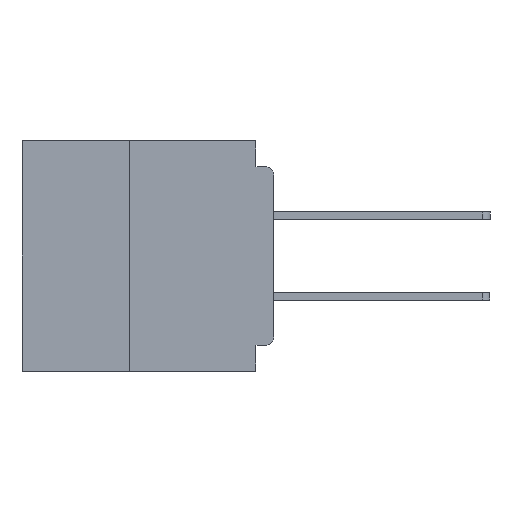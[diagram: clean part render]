
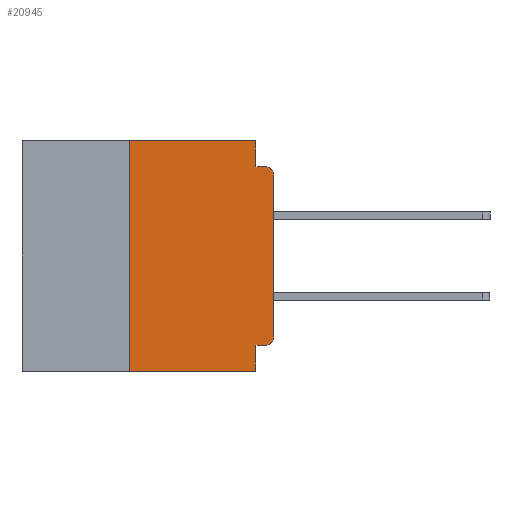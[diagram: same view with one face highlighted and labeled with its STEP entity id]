
A CAD part, left-side view. The second image highlights one B-rep face of the part: STEP entity #20945.
In plain terms, the highlighted planar face has unit normal (-1, 0, 0).
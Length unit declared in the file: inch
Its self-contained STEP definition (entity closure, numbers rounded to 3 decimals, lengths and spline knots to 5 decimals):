
#348 = CARTESIAN_POINT ( 'NONE',  ( 0., 0.25, -0.4 ) ) ;
#2660 = VECTOR ( 'NONE', #12221, 39.37008 ) ;
#2990 = EDGE_LOOP ( 'NONE', ( #30418, #12050, #26791, #27463, #31308, #37348, #7928, #6343, #39299, #18550 ) ) ;
#4067 = CARTESIAN_POINT ( 'NONE',  ( 0., 0., 0. ) ) ;
#4201 = AXIS2_PLACEMENT_3D ( 'NONE', #30078, #10522, #33375 ) ;
#5072 = CARTESIAN_POINT ( 'NONE',  ( 0., 0.437, 0. ) ) ;
#6161 = EDGE_CURVE ( 'NONE', #16101, #41000, #12043, .T. ) ;
#6162 = VECTOR ( 'NONE', #20634, 39.37008 ) ;
#6343 = ORIENTED_EDGE ( 'NONE', *, *, #12228, .F. ) ;
#6847 = VECTOR ( 'NONE', #16780, 39.37008 ) ;
#6880 = DIRECTION ( 'NONE',  ( 1., 0., 0. ) ) ;
#7031 = CARTESIAN_POINT ( 'NONE',  ( 0., 0.031, 0. ) ) ;
#7182 = EDGE_CURVE ( 'NONE', #24444, #38639, #15529, .T. ) ;
#7481 = VERTEX_POINT ( 'NONE', #21600 ) ;
#7928 = ORIENTED_EDGE ( 'NONE', *, *, #39443, .T. ) ;
#7967 = EDGE_CURVE ( 'NONE', #38639, #18185, #24130, .T. ) ;
#9271 = DIRECTION ( 'NONE',  ( -1., 0., 0. ) ) ;
#10268 = CIRCLE ( 'NONE', #4201, 0.015 ) ;
#10323 = DIRECTION ( 'NONE',  ( 0., 0., -1. ) ) ;
#10348 = LINE ( 'NONE', #31800, #2660 ) ;
#10522 = DIRECTION ( 'NONE',  ( -1., 0., 0. ) ) ;
#11561 = VERTEX_POINT ( 'NONE', #23038 ) ;
#12043 = LINE ( 'NONE', #14273, #30445 ) ;
#12050 = ORIENTED_EDGE ( 'NONE', *, *, #19523, .T. ) ;
#12221 = DIRECTION ( 'NONE',  ( 0., -1., 0. ) ) ;
#12228 = EDGE_CURVE ( 'NONE', #41000, #37942, #25846, .T. ) ;
#14273 = CARTESIAN_POINT ( 'NONE',  ( 0., 0., -0.355 ) ) ;
#15447 = VECTOR ( 'NONE', #27931, 39.37008 ) ;
#15529 = LINE ( 'NONE', #348, #6847 ) ;
#16101 = VERTEX_POINT ( 'NONE', #27505 ) ;
#16662 = AXIS2_PLACEMENT_3D ( 'NONE', #28851, #9271, #32152 ) ;
#16780 = DIRECTION ( 'NONE',  ( 0., 0., 1. ) ) ;
#16905 = VECTOR ( 'NONE', #10323, 39.37008 ) ;
#17351 = DIRECTION ( 'NONE',  ( 0., 0., 1. ) ) ;
#17408 = CARTESIAN_POINT ( 'NONE',  ( 0., 0.031, -0.355 ) ) ;
#18185 = VERTEX_POINT ( 'NONE', #19617 ) ;
#18550 = ORIENTED_EDGE ( 'NONE', *, *, #36495, .T. ) ;
#18929 = LINE ( 'NONE', #7031, #16905 ) ;
#19523 = EDGE_CURVE ( 'NONE', #22600, #7481, #39201, .T. ) ;
#19617 = CARTESIAN_POINT ( 'NONE',  ( 0., 0.031, 0. ) ) ;
#20634 = DIRECTION ( 'NONE',  ( 0., -1., 0. ) ) ;
#20945 = ADVANCED_FACE ( 'NONE', ( #34033 ), #36154, .F. ) ;
#21600 = CARTESIAN_POINT ( 'NONE',  ( 0., 0.015, -0.045 ) ) ;
#21919 = AXIS2_PLACEMENT_3D ( 'NONE', #39435, #6880, #29736 ) ;
#22600 = VERTEX_POINT ( 'NONE', #33522 ) ;
#23038 = CARTESIAN_POINT ( 'NONE',  ( 0., 0.031, -0.045 ) ) ;
#23089 = VERTEX_POINT ( 'NONE', #39040 ) ;
#23923 = CARTESIAN_POINT ( 'NONE',  ( 0., 0., -0.045 ) ) ;
#24130 = LINE ( 'NONE', #5072, #15447 ) ;
#24418 = CARTESIAN_POINT ( 'NONE',  ( 0., 0.25, 0. ) ) ;
#24444 = VERTEX_POINT ( 'NONE', #30228 ) ;
#25825 = LINE ( 'NONE', #4067, #41150 ) ;
#25846 = LINE ( 'NONE', #29852, #42188 ) ;
#26575 = DIRECTION ( 'NONE',  ( 0., 0., -1. ) ) ;
#26791 = ORIENTED_EDGE ( 'NONE', *, *, #36557, .F. ) ;
#27463 = ORIENTED_EDGE ( 'NONE', *, *, #40379, .F. ) ;
#27505 = CARTESIAN_POINT ( 'NONE',  ( 0., 0.015, -0.355 ) ) ;
#27931 = DIRECTION ( 'NONE',  ( 0., -1., 0. ) ) ;
#28851 = CARTESIAN_POINT ( 'NONE',  ( 0., 0.015, -0.06 ) ) ;
#29736 = DIRECTION ( 'NONE',  ( 0., 0., -1. ) ) ;
#29852 = CARTESIAN_POINT ( 'NONE',  ( 0., 0.031, -0.4 ) ) ;
#30078 = CARTESIAN_POINT ( 'NONE',  ( 0., 0.015, -0.34 ) ) ;
#30228 = CARTESIAN_POINT ( 'NONE',  ( 0., 0.25, -0.4 ) ) ;
#30418 = ORIENTED_EDGE ( 'NONE', *, *, #33875, .T. ) ;
#30445 = VECTOR ( 'NONE', #37121, 39.37008 ) ;
#31308 = ORIENTED_EDGE ( 'NONE', *, *, #7967, .F. ) ;
#31800 = CARTESIAN_POINT ( 'NONE',  ( 0., 0.437, -0.4 ) ) ;
#32152 = DIRECTION ( 'NONE',  ( 0., 0., -1. ) ) ;
#33375 = DIRECTION ( 'NONE',  ( 0., 0., -1. ) ) ;
#33522 = CARTESIAN_POINT ( 'NONE',  ( 0., 0., -0.06 ) ) ;
#33875 = EDGE_CURVE ( 'NONE', #23089, #22600, #25825, .T. ) ;
#34033 = FACE_OUTER_BOUND ( 'NONE', #2990, .T. ) ;
#36154 = PLANE ( 'NONE',  #21919 ) ;
#36495 = EDGE_CURVE ( 'NONE', #16101, #23089, #10268, .T. ) ;
#36557 = EDGE_CURVE ( 'NONE', #11561, #7481, #40900, .T. ) ;
#37121 = DIRECTION ( 'NONE',  ( 0., 1., 0. ) ) ;
#37328 = CARTESIAN_POINT ( 'NONE',  ( 0., 0.031, -0.4 ) ) ;
#37348 = ORIENTED_EDGE ( 'NONE', *, *, #7182, .F. ) ;
#37942 = VERTEX_POINT ( 'NONE', #37328 ) ;
#38639 = VERTEX_POINT ( 'NONE', #24418 ) ;
#39040 = CARTESIAN_POINT ( 'NONE',  ( 0., 0., -0.34 ) ) ;
#39201 = CIRCLE ( 'NONE', #16662, 0.015 ) ;
#39299 = ORIENTED_EDGE ( 'NONE', *, *, #6161, .F. ) ;
#39435 = CARTESIAN_POINT ( 'NONE',  ( 0., 0.437, 0. ) ) ;
#39443 = EDGE_CURVE ( 'NONE', #24444, #37942, #10348, .T. ) ;
#40379 = EDGE_CURVE ( 'NONE', #18185, #11561, #18929, .T. ) ;
#40900 = LINE ( 'NONE', #23923, #6162 ) ;
#41000 = VERTEX_POINT ( 'NONE', #17408 ) ;
#41150 = VECTOR ( 'NONE', #17351, 39.37008 ) ;
#42188 = VECTOR ( 'NONE', #26575, 39.37008 ) ;
